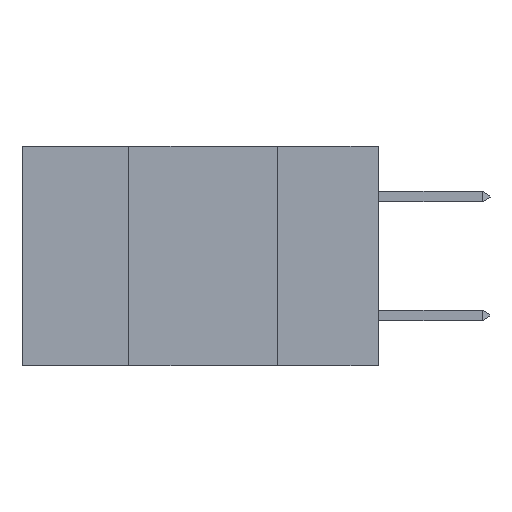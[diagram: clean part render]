
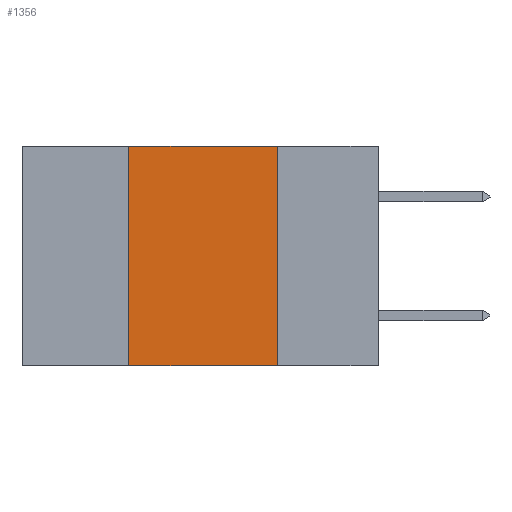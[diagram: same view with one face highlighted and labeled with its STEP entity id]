
A CAD part, left-side view. The second image highlights one B-rep face of the part: STEP entity #1356.
In plain terms, the highlighted planar face has unit normal (-1, 0, 0).
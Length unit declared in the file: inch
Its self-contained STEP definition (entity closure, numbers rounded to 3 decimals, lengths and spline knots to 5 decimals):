
#548 = LINE ( 'NONE', #10482, #4646 ) ;
#559 = FACE_OUTER_BOUND ( 'NONE', #2218, .T. ) ;
#1356 = ADVANCED_FACE ( 'NONE', ( #559 ), #3419, .F. ) ;
#1384 = LINE ( 'NONE', #8365, #2180 ) ;
#1500 = EDGE_CURVE ( 'NONE', #8186, #3978, #548, .T. ) ;
#1912 = CARTESIAN_POINT ( 'NONE',  ( 0., 0.6, 0. ) ) ;
#2129 = EDGE_CURVE ( 'NONE', #3575, #6917, #8996, .T. ) ;
#2154 = CARTESIAN_POINT ( 'NONE',  ( 0., 0.42, 0. ) ) ;
#2180 = VECTOR ( 'NONE', #3367, 39.37008 ) ;
#2203 = EDGE_CURVE ( 'NONE', #6917, #3978, #1384, .T. ) ;
#2218 = EDGE_LOOP ( 'NONE', ( #7964, #4364, #7026, #10420 ) ) ;
#2666 = DIRECTION ( 'NONE',  ( 0., 0., -1. ) ) ;
#3034 = CARTESIAN_POINT ( 'NONE',  ( 0., 0.17, -0.37 ) ) ;
#3367 = DIRECTION ( 'NONE',  ( 0., 0., -1. ) ) ;
#3419 = PLANE ( 'NONE',  #9653 ) ;
#3575 = VERTEX_POINT ( 'NONE', #2154 ) ;
#3768 = DIRECTION ( 'NONE',  ( 0., -1., 0. ) ) ;
#3978 = VERTEX_POINT ( 'NONE', #3034 ) ;
#4167 = VECTOR ( 'NONE', #8557, 39.37008 ) ;
#4364 = ORIENTED_EDGE ( 'NONE', *, *, #2129, .F. ) ;
#4646 = VECTOR ( 'NONE', #3768, 39.37008 ) ;
#4987 = DIRECTION ( 'NONE',  ( 0., -1., 0. ) ) ;
#5261 = CARTESIAN_POINT ( 'NONE',  ( 0., 0.42, 0. ) ) ;
#5833 = CARTESIAN_POINT ( 'NONE',  ( 0., 0.6, 0. ) ) ;
#6394 = LINE ( 'NONE', #5261, #4167 ) ;
#6917 = VERTEX_POINT ( 'NONE', #9613 ) ;
#7026 = ORIENTED_EDGE ( 'NONE', *, *, #9757, .F. ) ;
#7964 = ORIENTED_EDGE ( 'NONE', *, *, #2203, .F. ) ;
#8186 = VERTEX_POINT ( 'NONE', #9238 ) ;
#8365 = CARTESIAN_POINT ( 'NONE',  ( 0., 0.17, 0. ) ) ;
#8557 = DIRECTION ( 'NONE',  ( 0., 0., 1. ) ) ;
#8996 = LINE ( 'NONE', #5833, #10824 ) ;
#9238 = CARTESIAN_POINT ( 'NONE',  ( 0., 0.42, -0.37 ) ) ;
#9613 = CARTESIAN_POINT ( 'NONE',  ( 0., 0.17, 0. ) ) ;
#9653 = AXIS2_PLACEMENT_3D ( 'NONE', #1912, #10203, #2666 ) ;
#9757 = EDGE_CURVE ( 'NONE', #8186, #3575, #6394, .T. ) ;
#10203 = DIRECTION ( 'NONE',  ( 1., 0., 0. ) ) ;
#10420 = ORIENTED_EDGE ( 'NONE', *, *, #1500, .T. ) ;
#10482 = CARTESIAN_POINT ( 'NONE',  ( 0., 0.6, -0.37 ) ) ;
#10824 = VECTOR ( 'NONE', #4987, 39.37008 ) ;
